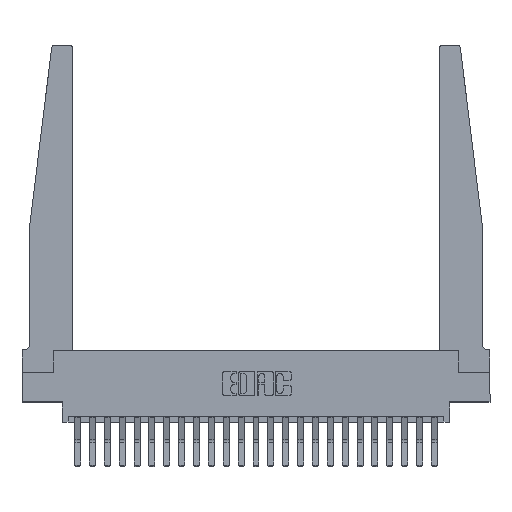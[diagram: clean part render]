
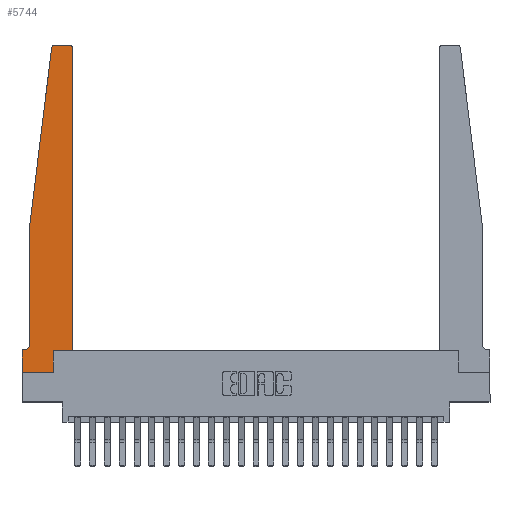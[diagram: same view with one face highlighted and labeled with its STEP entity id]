
A CAD part, top view. The second image highlights one B-rep face of the part: STEP entity #5744.
In plain terms, the highlighted planar face has unit normal (0, 0, 1).
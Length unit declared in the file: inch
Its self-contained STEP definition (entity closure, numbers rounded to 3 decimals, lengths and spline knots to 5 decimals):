
#220 = CARTESIAN_POINT ( 'NONE',  ( 0.425, 0.18, 0.37 ) ) ;
#262 = ORIENTED_EDGE ( 'NONE', *, *, #5990, .T. ) ;
#397 = DIRECTION ( 'NONE',  ( 0., 0., 1. ) ) ;
#577 = VECTOR ( 'NONE', #8659, 39.37008 ) ;
#620 = LINE ( 'NONE', #2680, #22562 ) ;
#785 = EDGE_CURVE ( 'NONE', #19041, #1182, #620, .T. ) ;
#836 = DIRECTION ( 'NONE',  ( -1., 0., 0. ) ) ;
#931 = EDGE_CURVE ( 'NONE', #15748, #15442, #1451, .T. ) ;
#1172 = CARTESIAN_POINT ( 'NONE',  ( 0.2605, 0.18, 0.37 ) ) ;
#1182 = VERTEX_POINT ( 'NONE', #7108 ) ;
#1451 = LINE ( 'NONE', #6804, #5445 ) ;
#1518 = EDGE_CURVE ( 'NONE', #5105, #5332, #4307, .T. ) ;
#1607 = CARTESIAN_POINT ( 'NONE',  ( 0.425, 2.72, 0.37 ) ) ;
#1785 = ORIENTED_EDGE ( 'NONE', *, *, #2707, .T. ) ;
#1906 = EDGE_CURVE ( 'NONE', #15733, #16744, #23408, .T. ) ;
#1998 = VECTOR ( 'NONE', #5259, 39.37008 ) ;
#2083 = VERTEX_POINT ( 'NONE', #11326 ) ;
#2680 = CARTESIAN_POINT ( 'NONE',  ( 0.065, 1.25, 0.37 ) ) ;
#2707 = EDGE_CURVE ( 'NONE', #12655, #15733, #9797, .T. ) ;
#2781 = DIRECTION ( 'NONE',  ( 0., 0., -1. ) ) ;
#3406 = CIRCLE ( 'NONE', #12340, 0.03 ) ;
#3417 = PLANE ( 'NONE',  #23515 ) ;
#4050 = CARTESIAN_POINT ( 'NONE',  ( 0.27653, 2.72, 0.37 ) ) ;
#4141 = LINE ( 'NONE', #20930, #6009 ) ;
#4221 = DIRECTION ( 'NONE',  ( 0., 1., 0. ) ) ;
#4302 = ORIENTED_EDGE ( 'NONE', *, *, #9496, .T. ) ;
#4307 = CIRCLE ( 'NONE', #17932, 0.03 ) ;
#4371 = ORIENTED_EDGE ( 'NONE', *, *, #11042, .T. ) ;
#4724 = DIRECTION ( 'NONE',  ( 0., 0., 1. ) ) ;
#5105 = VERTEX_POINT ( 'NONE', #1607 ) ;
#5143 = ORIENTED_EDGE ( 'NONE', *, *, #1906, .T. ) ;
#5259 = DIRECTION ( 'NONE',  ( -1., 0., 0. ) ) ;
#5307 = EDGE_LOOP ( 'NONE', ( #4371, #4302, #10167, #21804, #1785, #5143, #6023, #11376, #7544, #262, #9507, #22804 ) ) ;
#5332 = VERTEX_POINT ( 'NONE', #8647 ) ;
#5445 = VECTOR ( 'NONE', #12512, 39.37008 ) ;
#5744 = ADVANCED_FACE ( 'NONE', ( #20095 ), #3417, .T. ) ;
#5922 = LINE ( 'NONE', #9456, #15762 ) ;
#5990 = EDGE_CURVE ( 'NONE', #15442, #13850, #4141, .T. ) ;
#6009 = VECTOR ( 'NONE', #11551, 39.37008 ) ;
#6023 = ORIENTED_EDGE ( 'NONE', *, *, #16530, .T. ) ;
#6054 = LINE ( 'NONE', #19559, #20663 ) ;
#6072 = CARTESIAN_POINT ( 'NONE',  ( 0.015, 0.2375, 0.37 ) ) ;
#6225 = DIRECTION ( 'NONE',  ( 0., -1., 0. ) ) ;
#6804 = CARTESIAN_POINT ( 'NONE',  ( 0.2605, 0.18, 0.37 ) ) ;
#7108 = CARTESIAN_POINT ( 'NONE',  ( 0.065, 1.25, 0.37 ) ) ;
#7544 = ORIENTED_EDGE ( 'NONE', *, *, #931, .T. ) ;
#8647 = CARTESIAN_POINT ( 'NONE',  ( 0.395, 2.75, 0.37 ) ) ;
#8659 = DIRECTION ( 'NONE',  ( -1., 0., 0. ) ) ;
#8994 = CARTESIAN_POINT ( 'NONE',  ( 0.24675, 2.72367, 0.37 ) ) ;
#9024 = CARTESIAN_POINT ( 'NONE',  ( 0.065, 0.1875, 0.37 ) ) ;
#9193 = DIRECTION ( 'NONE',  ( 1., 0., 0. ) ) ;
#9456 = CARTESIAN_POINT ( 'NONE',  ( 0.425, 0.18, 0.37 ) ) ;
#9496 = EDGE_CURVE ( 'NONE', #2083, #19041, #3406, .T. ) ;
#9507 = ORIENTED_EDGE ( 'NONE', *, *, #20949, .T. ) ;
#9762 = DIRECTION ( 'NONE',  ( 1., 0., 0. ) ) ;
#9797 = CIRCLE ( 'NONE', #10201, 0.05 ) ;
#10153 = CARTESIAN_POINT ( 'NONE',  ( 0.2605, 0., 0.37 ) ) ;
#10167 = ORIENTED_EDGE ( 'NONE', *, *, #785, .T. ) ;
#10201 = AXIS2_PLACEMENT_3D ( 'NONE', #6072, #2781, #836 ) ;
#10326 = DIRECTION ( 'NONE',  ( 1., 0., 0. ) ) ;
#11042 = EDGE_CURVE ( 'NONE', #5332, #2083, #14147, .T. ) ;
#11326 = CARTESIAN_POINT ( 'NONE',  ( 0.27653, 2.75, 0.37 ) ) ;
#11376 = ORIENTED_EDGE ( 'NONE', *, *, #15603, .T. ) ;
#11551 = DIRECTION ( 'NONE',  ( 1., 0., 0. ) ) ;
#12340 = AXIS2_PLACEMENT_3D ( 'NONE', #4050, #397, #9762 ) ;
#12512 = DIRECTION ( 'NONE',  ( 0., 1., 0. ) ) ;
#12655 = VERTEX_POINT ( 'NONE', #14596 ) ;
#13144 = DIRECTION ( 'NONE',  ( 1., 0., 0. ) ) ;
#13543 = CARTESIAN_POINT ( 'NONE',  ( 0.065, 1.25, 0.37 ) ) ;
#13850 = VERTEX_POINT ( 'NONE', #220 ) ;
#13976 = CARTESIAN_POINT ( 'NONE',  ( 0.395, 2.72, 0.37 ) ) ;
#14147 = LINE ( 'NONE', #21790, #577 ) ;
#14596 = CARTESIAN_POINT ( 'NONE',  ( 0.065, 0.2375, 0.37 ) ) ;
#14671 = LINE ( 'NONE', #20506, #17914 ) ;
#15376 = LINE ( 'NONE', #13543, #19259 ) ;
#15399 = CARTESIAN_POINT ( 'NONE',  ( 0.015, 0.1875, 0.37 ) ) ;
#15442 = VERTEX_POINT ( 'NONE', #1172 ) ;
#15603 = EDGE_CURVE ( 'NONE', #17790, #15748, #14671, .T. ) ;
#15733 = VERTEX_POINT ( 'NONE', #15399 ) ;
#15748 = VERTEX_POINT ( 'NONE', #10153 ) ;
#15762 = VECTOR ( 'NONE', #4221, 39.37008 ) ;
#16530 = EDGE_CURVE ( 'NONE', #16744, #17790, #6054, .T. ) ;
#16630 = CARTESIAN_POINT ( 'NONE',  ( 0., 0., 0.37 ) ) ;
#16744 = VERTEX_POINT ( 'NONE', #21851 ) ;
#17790 = VERTEX_POINT ( 'NONE', #16630 ) ;
#17914 = VECTOR ( 'NONE', #9193, 39.37008 ) ;
#17932 = AXIS2_PLACEMENT_3D ( 'NONE', #13976, #4724, #10326 ) ;
#18268 = CARTESIAN_POINT ( 'NONE',  ( 0., 0.1875, 0.37 ) ) ;
#19041 = VERTEX_POINT ( 'NONE', #8994 ) ;
#19259 = VECTOR ( 'NONE', #6225, 39.37008 ) ;
#19355 = DIRECTION ( 'NONE',  ( -0.122, -0.992, 0. ) ) ;
#19559 = CARTESIAN_POINT ( 'NONE',  ( 0., 0., 0.37 ) ) ;
#20095 = FACE_OUTER_BOUND ( 'NONE', #5307, .T. ) ;
#20506 = CARTESIAN_POINT ( 'NONE',  ( 0., 0., 0.37 ) ) ;
#20663 = VECTOR ( 'NONE', #21016, 39.37008 ) ;
#20930 = CARTESIAN_POINT ( 'NONE',  ( 0.425, 0.18, 0.37 ) ) ;
#20949 = EDGE_CURVE ( 'NONE', #13850, #5105, #5922, .T. ) ;
#21016 = DIRECTION ( 'NONE',  ( 0., -1., 0. ) ) ;
#21790 = CARTESIAN_POINT ( 'NONE',  ( 0.25, 2.75, 0.37 ) ) ;
#21804 = ORIENTED_EDGE ( 'NONE', *, *, #23008, .T. ) ;
#21851 = CARTESIAN_POINT ( 'NONE',  ( 0., 0.1875, 0.37 ) ) ;
#22562 = VECTOR ( 'NONE', #19355, 39.37008 ) ;
#22804 = ORIENTED_EDGE ( 'NONE', *, *, #1518, .T. ) ;
#23008 = EDGE_CURVE ( 'NONE', #1182, #12655, #15376, .T. ) ;
#23408 = LINE ( 'NONE', #9024, #1998 ) ;
#23515 = AXIS2_PLACEMENT_3D ( 'NONE', #18268, #23857, #13144 ) ;
#23857 = DIRECTION ( 'NONE',  ( 0., 0., 1. ) ) ;
